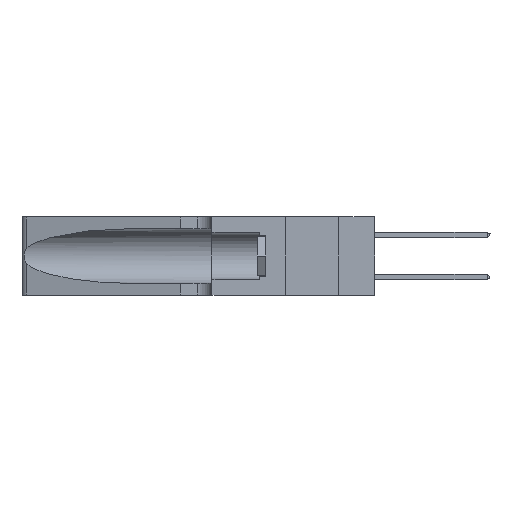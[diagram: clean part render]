
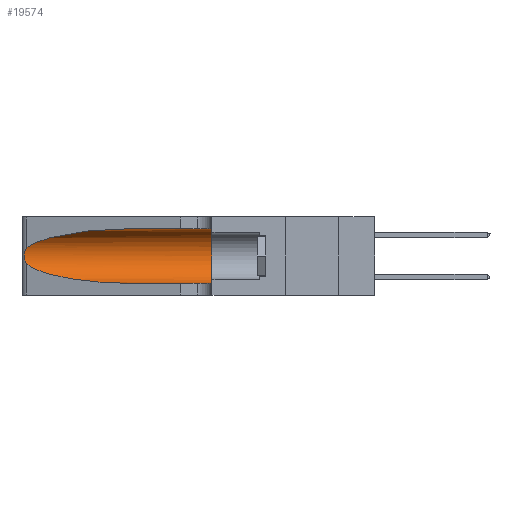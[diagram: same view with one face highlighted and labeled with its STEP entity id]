
A CAD part, left-side view. The second image highlights one B-rep face of the part: STEP entity #19574.
In plain terms, the highlighted cylindrical face has radius 3.308 mm (diameter 6.617 mm), a partial arc.
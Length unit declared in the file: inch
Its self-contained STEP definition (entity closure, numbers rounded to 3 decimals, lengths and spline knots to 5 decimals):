
#368 = CARTESIAN_POINT ( 'NONE',  ( 0.1305, 0.72297, 0.31525 ) ) ;
#636 = CARTESIAN_POINT ( 'NONE',  ( 0.1305, 0.72297, 0.31525 ) ) ;
#856 = CARTESIAN_POINT ( 'NONE',  ( 0.25487, 1.22718, 0.14631 ) ) ;
#1421 = ORIENTED_EDGE ( 'NONE', *, *, #9419, .F. ) ;
#1579 = CARTESIAN_POINT ( 'NONE',  ( 0.25787, 1.23484, 0.2124 ) ) ;
#2230 =( BOUNDED_CURVE ( )  B_SPLINE_CURVE ( 3, ( #368, #15411, #32870, #11134 ),
 .UNSPECIFIED., .F., .F. ) 
 B_SPLINE_CURVE_WITH_KNOTS ( ( 4, 4 ),
 ( 1.5708, 2.84003 ),
 .UNSPECIFIED. ) 
 CURVE ( )  GEOMETRIC_REPRESENTATION_ITEM ( )  RATIONAL_B_SPLINE_CURVE ( ( 1., 0.87, 0.87, 1. ) ) 
 REPRESENTATION_ITEM ( '' )  );
#2925 = CARTESIAN_POINT ( 'NONE',  ( 0.25487, 1.22718, 0.22369 ) ) ;
#3220 = CARTESIAN_POINT ( 'NONE',  ( 0.1305, 0.35, 0.31525 ) ) ;
#3277 = B_SPLINE_CURVE_WITH_KNOTS ( 'NONE', 3,
 ( #12476, #26041, #25916, #1579, #18065, #34220, #23323, #15209, #20816, #28996, #14960, #26428, #26166, #34448 ),
 .UNSPECIFIED., .F., .F.,
 ( 4, 2, 2, 2, 2, 2, 4 ),
 ( 0., 0.00027, 0.00053, 0.00107, 0.0016, 0.00187, 0.00214 ),
 .UNSPECIFIED. ) ;
#3415 = DIRECTION ( 'NONE',  ( 0., -1., 0. ) ) ;
#3513 = ORIENTED_EDGE ( 'NONE', *, *, #13210, .T. ) ;
#3682 = CARTESIAN_POINT ( 'NONE',  ( 0.1305, 0.35, 0.185 ) ) ;
#4222 = CARTESIAN_POINT ( 'NONE',  ( 0.1305, 0.72297, 0.05475 ) ) ;
#5585 = LINE ( 'NONE', #30611, #7285 ) ;
#6376 = CARTESIAN_POINT ( 'NONE',  ( 0.2373, 1.15595, 0.08982 ) ) ;
#7285 = VECTOR ( 'NONE', #3415, 39.37008 ) ;
#8339 = LINE ( 'NONE', #9534, #34716 ) ;
#9333 = AXIS2_PLACEMENT_3D ( 'NONE', #13941, #22502, #28154 ) ;
#9419 = EDGE_CURVE ( 'NONE', #15755, #26620, #8339, .T. ) ;
#9534 = CARTESIAN_POINT ( 'NONE',  ( 0.1305, 1.61858, 0.31525 ) ) ;
#10708 = EDGE_LOOP ( 'NONE', ( #31883, #34481, #3513, #11522, #16187, #1421 ) ) ;
#11134 = CARTESIAN_POINT ( 'NONE',  ( 0.25487, 1.22718, 0.22369 ) ) ;
#11522 = ORIENTED_EDGE ( 'NONE', *, *, #24081, .T. ) ;
#12476 = CARTESIAN_POINT ( 'NONE',  ( 0.25487, 1.22718, 0.22369 ) ) ;
#12679 = CARTESIAN_POINT ( 'NONE',  ( 0.1305, 0.35, 0.05475 ) ) ;
#13210 = EDGE_CURVE ( 'NONE', #15005, #27648, #19727, .T. ) ;
#13515 = CARTESIAN_POINT ( 'NONE',  ( 0.25487, 1.22718, 0.14631 ) ) ;
#13941 = CARTESIAN_POINT ( 'NONE',  ( 0.1305, 1.61858, 0.185 ) ) ;
#14033 = FACE_OUTER_BOUND ( 'NONE', #10708, .T. ) ;
#14960 = CARTESIAN_POINT ( 'NONE',  ( 0.25789, 1.23486, 0.15765 ) ) ;
#15005 = VERTEX_POINT ( 'NONE', #13515 ) ;
#15209 = CARTESIAN_POINT ( 'NONE',  ( 0.26075, 1.23896, 0.178 ) ) ;
#15411 = CARTESIAN_POINT ( 'NONE',  ( 0.18966, 0.96281, 0.31525 ) ) ;
#15739 = CYLINDRICAL_SURFACE ( 'NONE', #9333, 0.13025 ) ;
#15755 = VERTEX_POINT ( 'NONE', #636 ) ;
#16187 = ORIENTED_EDGE ( 'NONE', *, *, #31856, .F. ) ;
#16673 = CIRCLE ( 'NONE', #31029, 0.13025 ) ;
#18065 = CARTESIAN_POINT ( 'NONE',  ( 0.25854, 1.2359, 0.20912 ) ) ;
#18963 = DIRECTION ( 'NONE',  ( 0., -1., 0. ) ) ;
#19574 = ADVANCED_FACE ( 'NONE', ( #14033 ), #15739, .F. ) ;
#19720 = EDGE_CURVE ( 'NONE', #15755, #28450, #2230, .T. ) ;
#19727 =( BOUNDED_CURVE ( )  B_SPLINE_CURVE ( 3, ( #856, #6376, #25448, #4222 ),
 .UNSPECIFIED., .F., .F. ) 
 B_SPLINE_CURVE_WITH_KNOTS ( ( 4, 4 ),
 ( 3.44316, 4.71239 ),
 .UNSPECIFIED. ) 
 CURVE ( )  GEOMETRIC_REPRESENTATION_ITEM ( )  RATIONAL_B_SPLINE_CURVE ( ( 1., 0.87, 0.87, 1. ) ) 
 REPRESENTATION_ITEM ( '' )  );
#19988 = VERTEX_POINT ( 'NONE', #12679 ) ;
#20816 = CARTESIAN_POINT ( 'NONE',  ( 0.26017, 1.23833, 0.17102 ) ) ;
#22502 = DIRECTION ( 'NONE',  ( 0., -1., 0. ) ) ;
#23323 = CARTESIAN_POINT ( 'NONE',  ( 0.26075, 1.23896, 0.19203 ) ) ;
#24081 = EDGE_CURVE ( 'NONE', #27648, #19988, #5585, .T. ) ;
#24584 = DIRECTION ( 'NONE',  ( 0., 1., 0. ) ) ;
#25448 = CARTESIAN_POINT ( 'NONE',  ( 0.18966, 0.96281, 0.05475 ) ) ;
#25916 = CARTESIAN_POINT ( 'NONE',  ( 0.25639, 1.23184, 0.21858 ) ) ;
#26041 = CARTESIAN_POINT ( 'NONE',  ( 0.25555, 1.22994, 0.2215 ) ) ;
#26166 = CARTESIAN_POINT ( 'NONE',  ( 0.25555, 1.22993, 0.14849 ) ) ;
#26428 = CARTESIAN_POINT ( 'NONE',  ( 0.25639, 1.23186, 0.15144 ) ) ;
#26620 = VERTEX_POINT ( 'NONE', #3220 ) ;
#27648 = VERTEX_POINT ( 'NONE', #29755 ) ;
#28154 = DIRECTION ( 'NONE',  ( 0., 0., -1. ) ) ;
#28450 = VERTEX_POINT ( 'NONE', #2925 ) ;
#28996 = CARTESIAN_POINT ( 'NONE',  ( 0.25856, 1.23593, 0.16098 ) ) ;
#29755 = CARTESIAN_POINT ( 'NONE',  ( 0.1305, 0.72297, 0.05475 ) ) ;
#30611 = CARTESIAN_POINT ( 'NONE',  ( 0.1305, 1.61858, 0.05475 ) ) ;
#31029 = AXIS2_PLACEMENT_3D ( 'NONE', #3682, #24584, #32766 ) ;
#31856 = EDGE_CURVE ( 'NONE', #26620, #19988, #16673, .T. ) ;
#31883 = ORIENTED_EDGE ( 'NONE', *, *, #19720, .T. ) ;
#32766 = DIRECTION ( 'NONE',  ( 0., 0., 1. ) ) ;
#32860 = EDGE_CURVE ( 'NONE', #28450, #15005, #3277, .T. ) ;
#32870 = CARTESIAN_POINT ( 'NONE',  ( 0.2373, 1.15595, 0.28018 ) ) ;
#34220 = CARTESIAN_POINT ( 'NONE',  ( 0.26018, 1.23835, 0.19895 ) ) ;
#34448 = CARTESIAN_POINT ( 'NONE',  ( 0.25487, 1.22718, 0.14631 ) ) ;
#34481 = ORIENTED_EDGE ( 'NONE', *, *, #32860, .T. ) ;
#34716 = VECTOR ( 'NONE', #18963, 39.37008 ) ;
